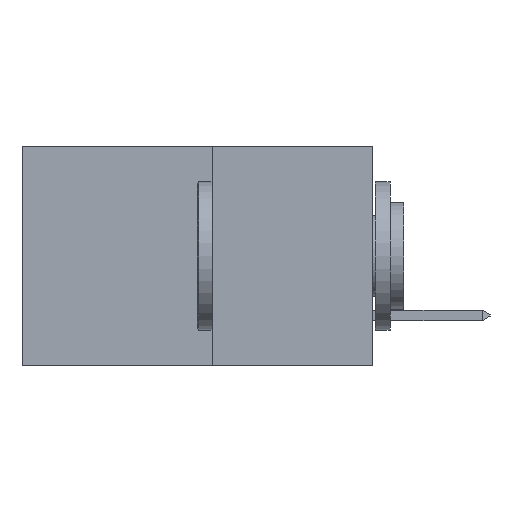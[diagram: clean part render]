
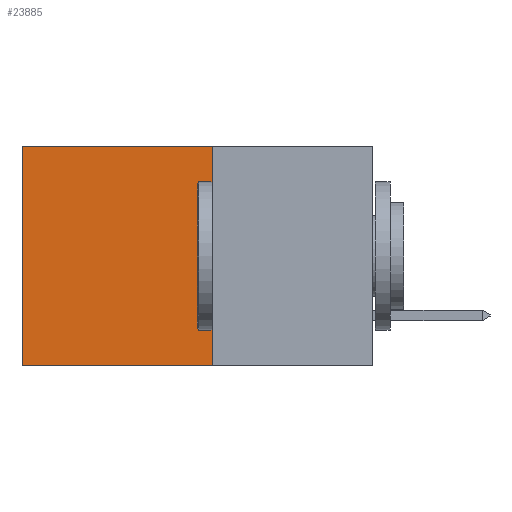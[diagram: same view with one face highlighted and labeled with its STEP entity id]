
A CAD part, left-side view. The second image highlights one B-rep face of the part: STEP entity #23885.
In plain terms, the highlighted planar face has unit normal (-1, 0, 0).
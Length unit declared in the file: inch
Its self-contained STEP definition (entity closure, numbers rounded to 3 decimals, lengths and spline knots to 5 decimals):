
#659 = VECTOR ( 'NONE', #14270, 39.37008 ) ;
#1134 = EDGE_CURVE ( 'NONE', #7637, #2767, #18645, .T. ) ;
#2581 = CARTESIAN_POINT ( 'NONE',  ( 0.277, 0.27, 0. ) ) ;
#2767 = VERTEX_POINT ( 'NONE', #15056 ) ;
#3979 = DIRECTION ( 'NONE',  ( 0., 0., -1. ) ) ;
#4689 = FACE_OUTER_BOUND ( 'NONE', #27951, .T. ) ;
#5886 = LINE ( 'NONE', #20601, #28320 ) ;
#6273 = EDGE_CURVE ( 'NONE', #14081, #22812, #20922, .T. ) ;
#6310 = CARTESIAN_POINT ( 'NONE',  ( 0.277, 0.27, -0.37 ) ) ;
#7637 = VERTEX_POINT ( 'NONE', #8410 ) ;
#7840 = LINE ( 'NONE', #12969, #13063 ) ;
#8410 = CARTESIAN_POINT ( 'NONE',  ( 0.277, 0.59, 0. ) ) ;
#8569 = AXIS2_PLACEMENT_3D ( 'NONE', #6310, #26488, #13058 ) ;
#8876 = CARTESIAN_POINT ( 'NONE',  ( 0.277, 0.59, -0.37 ) ) ;
#9114 = EDGE_CURVE ( 'NONE', #14081, #7637, #7840, .T. ) ;
#9326 = ORIENTED_EDGE ( 'NONE', *, *, #9114, .T. ) ;
#9501 = DIRECTION ( 'NONE',  ( 0., 1., 0. ) ) ;
#10699 = CARTESIAN_POINT ( 'NONE',  ( 0.277, 0.27, -0.37 ) ) ;
#12320 = EDGE_CURVE ( 'NONE', #22812, #2767, #5886, .T. ) ;
#12969 = CARTESIAN_POINT ( 'NONE',  ( 0.277, 0.27, 0. ) ) ;
#13058 = DIRECTION ( 'NONE',  ( 0., 0., -1. ) ) ;
#13063 = VECTOR ( 'NONE', #28626, 39.37008 ) ;
#13271 = ORIENTED_EDGE ( 'NONE', *, *, #6273, .F. ) ;
#14081 = VERTEX_POINT ( 'NONE', #2581 ) ;
#14270 = DIRECTION ( 'NONE',  ( 0., 0., -1. ) ) ;
#15056 = CARTESIAN_POINT ( 'NONE',  ( 0.277, 0.59, -0.37 ) ) ;
#17195 = ORIENTED_EDGE ( 'NONE', *, *, #1134, .T. ) ;
#18645 = LINE ( 'NONE', #8876, #659 ) ;
#19679 = PLANE ( 'NONE',  #8569 ) ;
#20554 = CARTESIAN_POINT ( 'NONE',  ( 0.277, 0.27, -0.37 ) ) ;
#20601 = CARTESIAN_POINT ( 'NONE',  ( 0.277, 0.27, -0.37 ) ) ;
#20922 = LINE ( 'NONE', #10699, #26937 ) ;
#21065 = ORIENTED_EDGE ( 'NONE', *, *, #12320, .F. ) ;
#22812 = VERTEX_POINT ( 'NONE', #20554 ) ;
#23885 = ADVANCED_FACE ( 'NONE', ( #4689 ), #19679, .F. ) ;
#26488 = DIRECTION ( 'NONE',  ( 1., 0., 0. ) ) ;
#26937 = VECTOR ( 'NONE', #3979, 39.37008 ) ;
#27951 = EDGE_LOOP ( 'NONE', ( #17195, #21065, #13271, #9326 ) ) ;
#28320 = VECTOR ( 'NONE', #9501, 39.37008 ) ;
#28626 = DIRECTION ( 'NONE',  ( 0., 1., 0. ) ) ;
